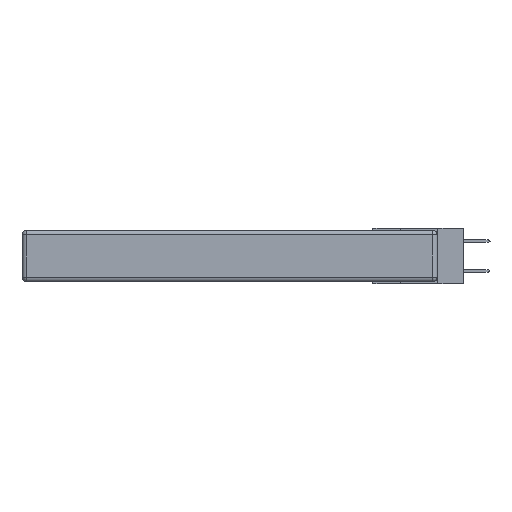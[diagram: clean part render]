
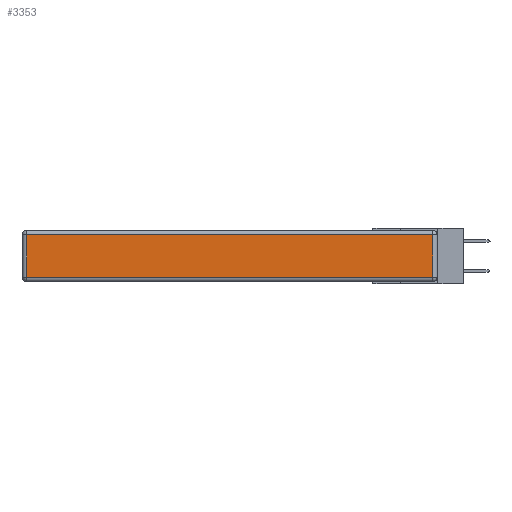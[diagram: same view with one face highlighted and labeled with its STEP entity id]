
A CAD part, left-side view. The second image highlights one B-rep face of the part: STEP entity #3353.
In plain terms, the highlighted planar face has unit normal (-1, 0, 0).
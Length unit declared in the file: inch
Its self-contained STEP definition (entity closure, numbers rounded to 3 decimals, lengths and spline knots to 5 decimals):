
#462 = DIRECTION ( 'NONE',  ( 0., 0., -1. ) ) ;
#681 = EDGE_CURVE ( 'NONE', #4353, #11393, #11976, .T. ) ;
#3353 = ADVANCED_FACE ( 'NONE', ( #5424 ), #7246, .T. ) ;
#4227 = EDGE_CURVE ( 'NONE', #7555, #8780, #12000, .T. ) ;
#4353 = VERTEX_POINT ( 'NONE', #14581 ) ;
#5424 = FACE_OUTER_BOUND ( 'NONE', #10682, .T. ) ;
#5474 = VECTOR ( 'NONE', #18612, 39.37008 ) ;
#5832 = ORIENTED_EDGE ( 'NONE', *, *, #681, .T. ) ;
#7246 = PLANE ( 'NONE',  #17481 ) ;
#7555 = VERTEX_POINT ( 'NONE', #14937 ) ;
#8020 = CARTESIAN_POINT ( 'NONE',  ( 0., 0.03, -0.343 ) ) ;
#8244 = CARTESIAN_POINT ( 'NONE',  ( 0., 0., -0.313 ) ) ;
#8426 = ORIENTED_EDGE ( 'NONE', *, *, #18896, .T. ) ;
#8780 = VERTEX_POINT ( 'NONE', #18967 ) ;
#9008 = ORIENTED_EDGE ( 'NONE', *, *, #4227, .T. ) ;
#9010 = VECTOR ( 'NONE', #14032, 39.37008 ) ;
#9487 = CARTESIAN_POINT ( 'NONE',  ( 0., 2.72, -0.03 ) ) ;
#10154 = CARTESIAN_POINT ( 'NONE',  ( 0., 2.75, -0.03 ) ) ;
#10172 = DIRECTION ( 'NONE',  ( 0., 0., 1. ) ) ;
#10682 = EDGE_LOOP ( 'NONE', ( #9008, #8426, #5832, #12725 ) ) ;
#11393 = VERTEX_POINT ( 'NONE', #9487 ) ;
#11411 = EDGE_CURVE ( 'NONE', #11393, #7555, #16476, .T. ) ;
#11781 = DIRECTION ( 'NONE',  ( 0., 1., 0. ) ) ;
#11802 = LINE ( 'NONE', #8020, #9010 ) ;
#11976 = LINE ( 'NONE', #10154, #14314 ) ;
#12000 = LINE ( 'NONE', #8244, #5474 ) ;
#12348 = CARTESIAN_POINT ( 'NONE',  ( 0., 2.72, -0.343 ) ) ;
#12725 = ORIENTED_EDGE ( 'NONE', *, *, #11411, .T. ) ;
#13412 = VECTOR ( 'NONE', #462, 39.37008 ) ;
#14032 = DIRECTION ( 'NONE',  ( 0., 0., 1. ) ) ;
#14314 = VECTOR ( 'NONE', #11781, 39.37008 ) ;
#14581 = CARTESIAN_POINT ( 'NONE',  ( 0., 0.03, -0.03 ) ) ;
#14937 = CARTESIAN_POINT ( 'NONE',  ( 0., 2.72, -0.313 ) ) ;
#16016 = DIRECTION ( 'NONE',  ( -1., 0., 0. ) ) ;
#16476 = LINE ( 'NONE', #12348, #13412 ) ;
#17481 = AXIS2_PLACEMENT_3D ( 'NONE', #17794, #16016, #10172 ) ;
#17794 = CARTESIAN_POINT ( 'NONE',  ( 0., 0., -0.343 ) ) ;
#18612 = DIRECTION ( 'NONE',  ( 0., -1., 0. ) ) ;
#18896 = EDGE_CURVE ( 'NONE', #8780, #4353, #11802, .T. ) ;
#18967 = CARTESIAN_POINT ( 'NONE',  ( 0., 0.03, -0.313 ) ) ;
